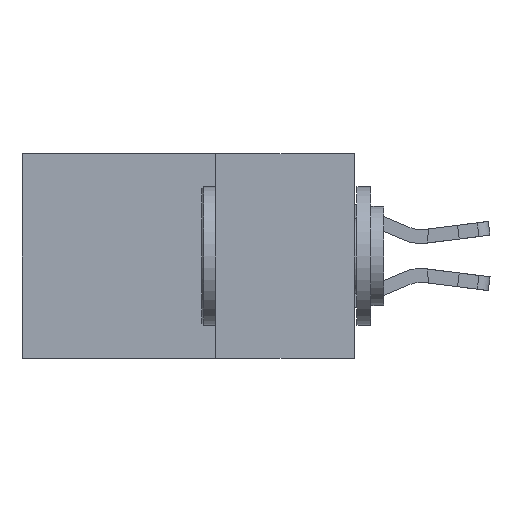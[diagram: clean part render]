
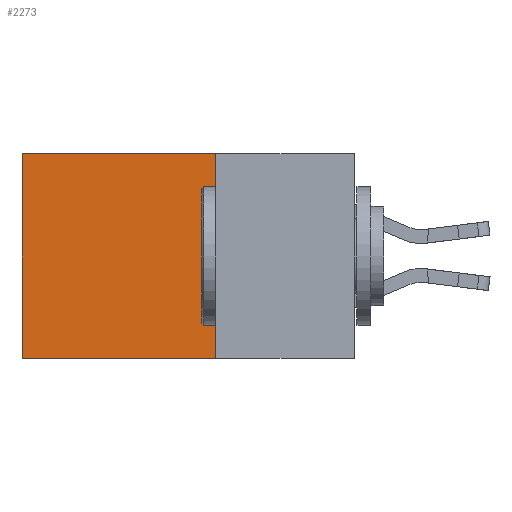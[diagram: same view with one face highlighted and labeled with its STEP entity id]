
A CAD part, left-side view. The second image highlights one B-rep face of the part: STEP entity #2273.
In plain terms, the highlighted planar face has unit normal (-1, 0, 0).
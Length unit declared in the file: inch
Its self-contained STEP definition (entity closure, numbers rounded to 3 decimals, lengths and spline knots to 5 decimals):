
#127 = CARTESIAN_POINT ( 'NONE',  ( 0.2615, 0.25, -0.37 ) ) ;
#165 = VECTOR ( 'NONE', #1654, 39.37008 ) ;
#208 = CARTESIAN_POINT ( 'NONE',  ( 0.2615, 0.25, -0.37 ) ) ;
#294 = PLANE ( 'NONE',  #13197 ) ;
#636 = LINE ( 'NONE', #127, #165 ) ;
#1654 = DIRECTION ( 'NONE',  ( 0., 0., -1. ) ) ;
#2273 = ADVANCED_FACE ( 'NONE', ( #3749 ), #294, .F. ) ;
#2314 = EDGE_LOOP ( 'NONE', ( #9691, #19050, #14136, #6724 ) ) ;
#2729 = CARTESIAN_POINT ( 'NONE',  ( 0.2615, 0.25, -0.37 ) ) ;
#3749 = FACE_OUTER_BOUND ( 'NONE', #2314, .T. ) ;
#3980 = VECTOR ( 'NONE', #4258, 39.37008 ) ;
#4258 = DIRECTION ( 'NONE',  ( 0., 1., 0. ) ) ;
#4950 = DIRECTION ( 'NONE',  ( 0., 0., -1. ) ) ;
#6491 = CARTESIAN_POINT ( 'NONE',  ( 0.2615, 0.25, 0. ) ) ;
#6724 = ORIENTED_EDGE ( 'NONE', *, *, #19271, .T. ) ;
#7261 = LINE ( 'NONE', #6491, #18976 ) ;
#7482 = EDGE_CURVE ( 'NONE', #18244, #14415, #18722, .T. ) ;
#7485 = DIRECTION ( 'NONE',  ( 0., 0., -1. ) ) ;
#8897 = VERTEX_POINT ( 'NONE', #208 ) ;
#9691 = ORIENTED_EDGE ( 'NONE', *, *, #7482, .T. ) ;
#12149 = LINE ( 'NONE', #2729, #3980 ) ;
#12649 = DIRECTION ( 'NONE',  ( 0., 1., 0. ) ) ;
#13197 = AXIS2_PLACEMENT_3D ( 'NONE', #18678, #14142, #4950 ) ;
#13617 = VERTEX_POINT ( 'NONE', #19673 ) ;
#14136 = ORIENTED_EDGE ( 'NONE', *, *, #15717, .F. ) ;
#14142 = DIRECTION ( 'NONE',  ( 1., 0., 0. ) ) ;
#14188 = VECTOR ( 'NONE', #7485, 39.37008 ) ;
#14415 = VERTEX_POINT ( 'NONE', #15325 ) ;
#14819 = EDGE_CURVE ( 'NONE', #8897, #14415, #12149, .T. ) ;
#15176 = CARTESIAN_POINT ( 'NONE',  ( 0.2615, 0.6, 0. ) ) ;
#15325 = CARTESIAN_POINT ( 'NONE',  ( 0.2615, 0.6, -0.37 ) ) ;
#15717 = EDGE_CURVE ( 'NONE', #13617, #8897, #636, .T. ) ;
#18183 = CARTESIAN_POINT ( 'NONE',  ( 0.2615, 0.6, -0.37 ) ) ;
#18244 = VERTEX_POINT ( 'NONE', #15176 ) ;
#18678 = CARTESIAN_POINT ( 'NONE',  ( 0.2615, 0.25, -0.37 ) ) ;
#18722 = LINE ( 'NONE', #18183, #14188 ) ;
#18976 = VECTOR ( 'NONE', #12649, 39.37008 ) ;
#19050 = ORIENTED_EDGE ( 'NONE', *, *, #14819, .F. ) ;
#19271 = EDGE_CURVE ( 'NONE', #13617, #18244, #7261, .T. ) ;
#19673 = CARTESIAN_POINT ( 'NONE',  ( 0.2615, 0.25, 0. ) ) ;
